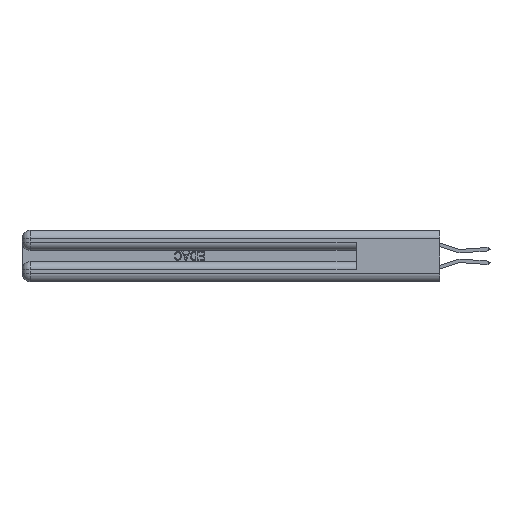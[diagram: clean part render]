
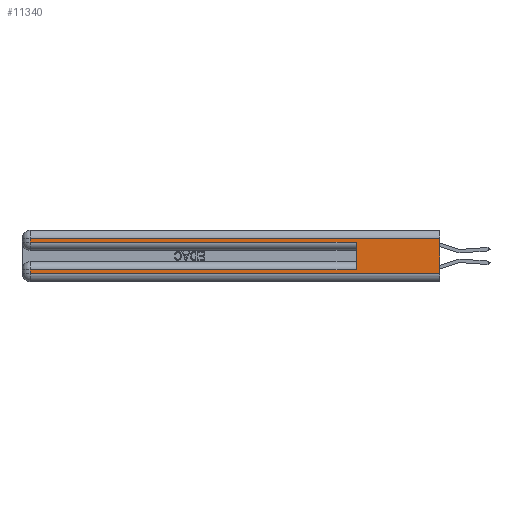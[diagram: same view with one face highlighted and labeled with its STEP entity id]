
A CAD part, left-side view. The second image highlights one B-rep face of the part: STEP entity #11340.
In plain terms, the highlighted planar face has unit normal (-1, 0, 0).
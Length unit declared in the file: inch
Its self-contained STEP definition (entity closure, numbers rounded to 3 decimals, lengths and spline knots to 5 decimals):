
#447 = CARTESIAN_POINT ( 'NONE',  ( 0., 0.6, 0.085 ) ) ;
#1267 = DIRECTION ( 'NONE',  ( 0., -1., 0. ) ) ;
#1681 = VERTEX_POINT ( 'NONE', #35657 ) ;
#3132 = EDGE_CURVE ( 'NONE', #1681, #7416, #34768, .T. ) ;
#3213 = VECTOR ( 'NONE', #25331, 39.37008 ) ;
#3884 = VERTEX_POINT ( 'NONE', #29435 ) ;
#4131 = VECTOR ( 'NONE', #13320, 39.37008 ) ;
#4539 = CARTESIAN_POINT ( 'NONE',  ( 0., 0., 0.31 ) ) ;
#5185 = ORIENTED_EDGE ( 'NONE', *, *, #20733, .T. ) ;
#5836 = CARTESIAN_POINT ( 'NONE',  ( 0., 0., 0.06 ) ) ;
#6470 = VERTEX_POINT ( 'NONE', #12219 ) ;
#6706 = ORIENTED_EDGE ( 'NONE', *, *, #25039, .T. ) ;
#6983 = VERTEX_POINT ( 'NONE', #20090 ) ;
#7401 = EDGE_CURVE ( 'NONE', #6983, #3884, #29130, .T. ) ;
#7416 = VERTEX_POINT ( 'NONE', #37010 ) ;
#7760 = CARTESIAN_POINT ( 'NONE',  ( 0., 0.6, 0.145 ) ) ;
#8752 = CARTESIAN_POINT ( 'NONE',  ( 0., 2.94, 0.37 ) ) ;
#8996 = DIRECTION ( 'NONE',  ( 0., 0., -1. ) ) ;
#10038 = LINE ( 'NONE', #34157, #32331 ) ;
#10761 = CARTESIAN_POINT ( 'NONE',  ( 0., 0., 0.37 ) ) ;
#10951 = LINE ( 'NONE', #7760, #3213 ) ;
#11173 = ORIENTED_EDGE ( 'NONE', *, *, #15673, .T. ) ;
#11340 = ADVANCED_FACE ( 'NONE', ( #11432 ), #29616, .F. ) ;
#11427 = ORIENTED_EDGE ( 'NONE', *, *, #7401, .F. ) ;
#11432 = FACE_OUTER_BOUND ( 'NONE', #27917, .T. ) ;
#12097 = DIRECTION ( 'NONE',  ( 0., -1., 0. ) ) ;
#12165 = DIRECTION ( 'NONE',  ( 1., 0., 0. ) ) ;
#12219 = CARTESIAN_POINT ( 'NONE',  ( 0., 2.94, 0.31 ) ) ;
#13318 = AXIS2_PLACEMENT_3D ( 'NONE', #26705, #12165, #32514 ) ;
#13320 = DIRECTION ( 'NONE',  ( 0., 1., 0. ) ) ;
#15673 = EDGE_CURVE ( 'NONE', #6470, #33946, #28417, .T. ) ;
#17135 = CARTESIAN_POINT ( 'NONE',  ( 0., 0.6, 0.285 ) ) ;
#17532 = CARTESIAN_POINT ( 'NONE',  ( 0., 2.94, 0.285 ) ) ;
#18634 = VERTEX_POINT ( 'NONE', #17135 ) ;
#20090 = CARTESIAN_POINT ( 'NONE',  ( 0., 0., 0.31 ) ) ;
#20188 = EDGE_CURVE ( 'NONE', #33946, #18634, #23499, .T. ) ;
#20733 = EDGE_CURVE ( 'NONE', #7416, #3884, #35195, .T. ) ;
#23499 = LINE ( 'NONE', #24573, #31223 ) ;
#23522 = CARTESIAN_POINT ( 'NONE',  ( 0., 2.94, 0.37 ) ) ;
#24573 = CARTESIAN_POINT ( 'NONE',  ( 0., 0., 0.285 ) ) ;
#25039 = EDGE_CURVE ( 'NONE', #6983, #6470, #35024, .T. ) ;
#25331 = DIRECTION ( 'NONE',  ( 0., 0., 1. ) ) ;
#25422 = VERTEX_POINT ( 'NONE', #447 ) ;
#26705 = CARTESIAN_POINT ( 'NONE',  ( 0., 0., 0.37 ) ) ;
#27535 = VECTOR ( 'NONE', #12097, 39.37008 ) ;
#27917 = EDGE_LOOP ( 'NONE', ( #11427, #6706, #11173, #31298, #37181, #28637, #30053, #5185 ) ) ;
#28035 = VECTOR ( 'NONE', #32019, 39.37008 ) ;
#28226 = VECTOR ( 'NONE', #31133, 39.37008 ) ;
#28254 = DIRECTION ( 'NONE',  ( 0., 1., 0. ) ) ;
#28417 = LINE ( 'NONE', #23522, #36954 ) ;
#28637 = ORIENTED_EDGE ( 'NONE', *, *, #30048, .T. ) ;
#29130 = LINE ( 'NONE', #10761, #28226 ) ;
#29435 = CARTESIAN_POINT ( 'NONE',  ( 0., 0., 0.06 ) ) ;
#29616 = PLANE ( 'NONE',  #13318 ) ;
#29992 = EDGE_CURVE ( 'NONE', #25422, #18634, #10951, .T. ) ;
#30048 = EDGE_CURVE ( 'NONE', #25422, #1681, #10038, .T. ) ;
#30053 = ORIENTED_EDGE ( 'NONE', *, *, #3132, .T. ) ;
#31133 = DIRECTION ( 'NONE',  ( 0., 0., -1. ) ) ;
#31223 = VECTOR ( 'NONE', #1267, 39.37008 ) ;
#31298 = ORIENTED_EDGE ( 'NONE', *, *, #20188, .T. ) ;
#32019 = DIRECTION ( 'NONE',  ( 0., 0., -1. ) ) ;
#32331 = VECTOR ( 'NONE', #28254, 39.37008 ) ;
#32514 = DIRECTION ( 'NONE',  ( 0., 0., -1. ) ) ;
#33946 = VERTEX_POINT ( 'NONE', #17532 ) ;
#34157 = CARTESIAN_POINT ( 'NONE',  ( 0., 0., 0.085 ) ) ;
#34768 = LINE ( 'NONE', #8752, #28035 ) ;
#35024 = LINE ( 'NONE', #4539, #4131 ) ;
#35195 = LINE ( 'NONE', #5836, #27535 ) ;
#35657 = CARTESIAN_POINT ( 'NONE',  ( 0., 2.94, 0.085 ) ) ;
#36954 = VECTOR ( 'NONE', #8996, 39.37008 ) ;
#37010 = CARTESIAN_POINT ( 'NONE',  ( 0., 2.94, 0.06 ) ) ;
#37181 = ORIENTED_EDGE ( 'NONE', *, *, #29992, .F. ) ;
